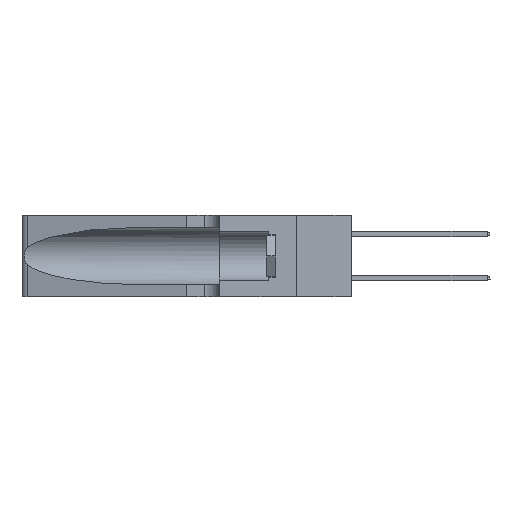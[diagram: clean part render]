
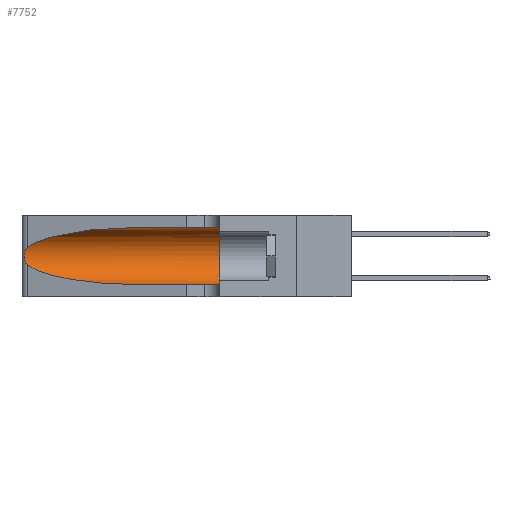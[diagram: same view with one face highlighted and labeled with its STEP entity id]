
A CAD part, left-side view. The second image highlights one B-rep face of the part: STEP entity #7752.
In plain terms, the highlighted cylindrical face has radius 3.308 mm (diameter 6.617 mm), a partial arc.
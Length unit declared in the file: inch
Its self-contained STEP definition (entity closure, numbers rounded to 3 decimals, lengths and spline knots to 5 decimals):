
#334 = ORIENTED_EDGE ( 'NONE', *, *, #12280, .T. ) ;
#898 = ORIENTED_EDGE ( 'NONE', *, *, #13319, .F. ) ;
#2189 = EDGE_CURVE ( 'NONE', #26192, #37116, #40575, .T. ) ;
#2415 = CARTESIAN_POINT ( 'NONE',  ( 0.1305, 0.35, 0.31525 ) ) ;
#2449 = CARTESIAN_POINT ( 'NONE',  ( 0.25487, 1.22718, 0.14631 ) ) ;
#2757 = CARTESIAN_POINT ( 'NONE',  ( 0.25639, 1.23186, 0.15144 ) ) ;
#3691 = CARTESIAN_POINT ( 'NONE',  ( 0.1305, 1.61858, 0.31525 ) ) ;
#4842 = EDGE_CURVE ( 'NONE', #37116, #9686, #9344, .T. ) ;
#6244 = CARTESIAN_POINT ( 'NONE',  ( 0.25639, 1.23184, 0.21858 ) ) ;
#6549 = VECTOR ( 'NONE', #14861, 39.37008 ) ;
#6705 = CARTESIAN_POINT ( 'NONE',  ( 0.25555, 1.22994, 0.2215 ) ) ;
#6832 = ORIENTED_EDGE ( 'NONE', *, *, #21851, .F. ) ;
#7166 = LINE ( 'NONE', #3691, #36254 ) ;
#7752 = ADVANCED_FACE ( 'NONE', ( #40360 ), #28696, .F. ) ;
#7786 = ORIENTED_EDGE ( 'NONE', *, *, #2189, .T. ) ;
#7872 = AXIS2_PLACEMENT_3D ( 'NONE', #29184, #11330, #28883 ) ;
#7879 = CARTESIAN_POINT ( 'NONE',  ( 0.1305, 0.72297, 0.05475 ) ) ;
#7991 = DIRECTION ( 'NONE',  ( 0., -1., 0. ) ) ;
#8655 = ORIENTED_EDGE ( 'NONE', *, *, #4842, .T. ) ;
#9234 = VERTEX_POINT ( 'NONE', #23329 ) ;
#9344 = LINE ( 'NONE', #32553, #6549 ) ;
#9686 = VERTEX_POINT ( 'NONE', #40447 ) ;
#9812 = CIRCLE ( 'NONE', #7872, 0.13025 ) ;
#9815 = ORIENTED_EDGE ( 'NONE', *, *, #24869, .T. ) ;
#9834 = CARTESIAN_POINT ( 'NONE',  ( 0.25555, 1.22993, 0.14849 ) ) ;
#11330 = DIRECTION ( 'NONE',  ( 0., 1., 0. ) ) ;
#12280 = EDGE_CURVE ( 'NONE', #9234, #26192, #42564, .T. ) ;
#13319 = EDGE_CURVE ( 'NONE', #31252, #25609, #7166, .T. ) ;
#13583 = CARTESIAN_POINT ( 'NONE',  ( 0.25787, 1.23484, 0.2124 ) ) ;
#13738 = CARTESIAN_POINT ( 'NONE',  ( 0.25487, 1.22718, 0.22369 ) ) ;
#14404 = CARTESIAN_POINT ( 'NONE',  ( 0.25487, 1.22718, 0.14631 ) ) ;
#14861 = DIRECTION ( 'NONE',  ( 0., -1., 0. ) ) ;
#15022 = CARTESIAN_POINT ( 'NONE',  ( 0.1305, 1.61858, 0.185 ) ) ;
#15558 = CARTESIAN_POINT ( 'NONE',  ( 0.25487, 1.22718, 0.22369 ) ) ;
#17336 = CARTESIAN_POINT ( 'NONE',  ( 0.26018, 1.23835, 0.19895 ) ) ;
#17843 = CARTESIAN_POINT ( 'NONE',  ( 0.1305, 0.72297, 0.05475 ) ) ;
#18445 = DIRECTION ( 'NONE',  ( 0., 0., -1. ) ) ;
#18662 = CARTESIAN_POINT ( 'NONE',  ( 0.1305, 0.72297, 0.31525 ) ) ;
#20963 = CARTESIAN_POINT ( 'NONE',  ( 0.25789, 1.23486, 0.15765 ) ) ;
#21337 = CARTESIAN_POINT ( 'NONE',  ( 0.18966, 0.96281, 0.05475 ) ) ;
#21851 = EDGE_CURVE ( 'NONE', #25609, #9686, #9812, .T. ) ;
#22603 =( BOUNDED_CURVE ( )  B_SPLINE_CURVE ( 3, ( #18662, #25757, #29339, #15558 ),
 .UNSPECIFIED., .F., .T. ) 
 B_SPLINE_CURVE_WITH_KNOTS ( ( 4, 4 ),
 ( 1.5708, 2.84003 ),
 .UNSPECIFIED. ) 
 CURVE ( )  GEOMETRIC_REPRESENTATION_ITEM ( )  RATIONAL_B_SPLINE_CURVE ( ( 1., 0.87, 0.87, 1. ) ) 
 REPRESENTATION_ITEM ( '' )  );
#23329 = CARTESIAN_POINT ( 'NONE',  ( 0.25487, 1.22718, 0.22369 ) ) ;
#23939 = CARTESIAN_POINT ( 'NONE',  ( 0.25856, 1.23593, 0.16098 ) ) ;
#24869 = EDGE_CURVE ( 'NONE', #31252, #9234, #22603, .T. ) ;
#25609 = VERTEX_POINT ( 'NONE', #2415 ) ;
#25646 = DIRECTION ( 'NONE',  ( 0., -1., 0. ) ) ;
#25757 = CARTESIAN_POINT ( 'NONE',  ( 0.18966, 0.96281, 0.31525 ) ) ;
#26192 = VERTEX_POINT ( 'NONE', #34445 ) ;
#27556 = CARTESIAN_POINT ( 'NONE',  ( 0.26075, 1.23896, 0.19203 ) ) ;
#27701 = CARTESIAN_POINT ( 'NONE',  ( 0.26017, 1.23833, 0.17102 ) ) ;
#28696 = CYLINDRICAL_SURFACE ( 'NONE', #30085, 0.13025 ) ;
#28883 = DIRECTION ( 'NONE',  ( 0., 0., 1. ) ) ;
#29184 = CARTESIAN_POINT ( 'NONE',  ( 0.1305, 0.35, 0.185 ) ) ;
#29339 = CARTESIAN_POINT ( 'NONE',  ( 0.2373, 1.15595, 0.28018 ) ) ;
#30085 = AXIS2_PLACEMENT_3D ( 'NONE', #15022, #7991, #18445 ) ;
#31252 = VERTEX_POINT ( 'NONE', #31686 ) ;
#31686 = CARTESIAN_POINT ( 'NONE',  ( 0.1305, 0.72297, 0.31525 ) ) ;
#32553 = CARTESIAN_POINT ( 'NONE',  ( 0.1305, 1.61858, 0.05475 ) ) ;
#34445 = CARTESIAN_POINT ( 'NONE',  ( 0.25487, 1.22718, 0.14631 ) ) ;
#34673 = CARTESIAN_POINT ( 'NONE',  ( 0.25854, 1.2359, 0.20912 ) ) ;
#34968 = CARTESIAN_POINT ( 'NONE',  ( 0.26075, 1.23896, 0.178 ) ) ;
#36254 = VECTOR ( 'NONE', #25646, 39.37008 ) ;
#37116 = VERTEX_POINT ( 'NONE', #7879 ) ;
#39114 = EDGE_LOOP ( 'NONE', ( #9815, #334, #7786, #8655, #6832, #898 ) ) ;
#40360 = FACE_OUTER_BOUND ( 'NONE', #39114, .T. ) ;
#40447 = CARTESIAN_POINT ( 'NONE',  ( 0.1305, 0.35, 0.05475 ) ) ;
#40575 =( BOUNDED_CURVE ( )  B_SPLINE_CURVE ( 3, ( #14404, #46011, #21337, #17843 ),
 .UNSPECIFIED., .F., .T. ) 
 B_SPLINE_CURVE_WITH_KNOTS ( ( 4, 4 ),
 ( 3.44316, 4.71239 ),
 .UNSPECIFIED. ) 
 CURVE ( )  GEOMETRIC_REPRESENTATION_ITEM ( )  RATIONAL_B_SPLINE_CURVE ( ( 1., 0.87, 0.87, 1. ) ) 
 REPRESENTATION_ITEM ( '' )  );
#42564 = B_SPLINE_CURVE_WITH_KNOTS ( 'NONE', 3,
 ( #13738, #6705, #6244, #13583, #34673, #17336, #27556, #34968, #27701, #23939, #20963, #2757, #9834, #2449 ),
 .UNSPECIFIED., .F., .F.,
 ( 4, 2, 2, 2, 2, 2, 4 ),
 ( 0., 0.00027, 0.00053, 0.00107, 0.0016, 0.00187, 0.00214 ),
 .UNSPECIFIED. ) ;
#46011 = CARTESIAN_POINT ( 'NONE',  ( 0.2373, 1.15595, 0.08982 ) ) ;
